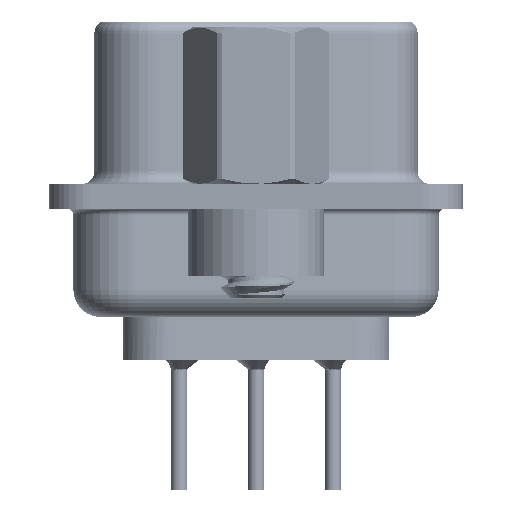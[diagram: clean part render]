
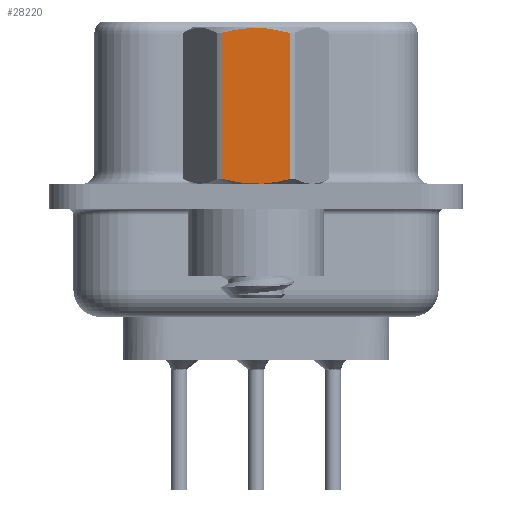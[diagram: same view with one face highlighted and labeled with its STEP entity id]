
A CAD part, left-side view. The second image highlights one B-rep face of the part: STEP entity #28220.
In plain terms, the highlighted planar face has unit normal (-1, 0, 0).
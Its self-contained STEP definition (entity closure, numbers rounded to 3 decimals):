
#46 = DIRECTION ( 'NONE',  ( 0., 0., -1. ) ) ;
#1586 = CARTESIAN_POINT ( 'NONE',  ( -2.381, 0.215, 6.232 ) ) ;
#3322 = VERTEX_POINT ( 'NONE', #21948 ) ;
#4261 = CARTESIAN_POINT ( 'NONE',  ( -2.381, 0.215, 0.468 ) ) ;
#6745 = CARTESIAN_POINT ( 'NONE',  ( -2.381, 1.273, 0.652 ) ) ;
#6927 = ORIENTED_EDGE ( 'NONE', *, *, #16355, .T. ) ;
#8190 = CARTESIAN_POINT ( 'NONE',  ( -2.381, 1.273, 6.048 ) ) ;
#8741 = LINE ( 'NONE', #14932, #22452 ) ;
#8798 = CARTESIAN_POINT ( 'NONE',  ( -2.381, 0.853, 6.151 ) ) ;
#10250 = CARTESIAN_POINT ( 'NONE',  ( -2.381, -1.273, 0.652 ) ) ;
#10459 = CARTESIAN_POINT ( 'NONE',  ( -2.381, -0.432, 0.485 ) ) ;
#10868 = CARTESIAN_POINT ( 'NONE',  ( -2.381, 1.065, 0.596 ) ) ;
#11129 = B_SPLINE_CURVE_WITH_KNOTS ( 'NONE', 3,
 ( #6745, #10868, #26337, #38489, #4261, #26128, #10459, #34998, #19337, #10250 ),
 .UNSPECIFIED., .F., .F.,
 ( 4, 2, 2, 2, 4 ),
 ( 0.003, 0.003, 0.004, 0.004, 0.005 ),
 .UNSPECIFIED. ) ;
#11699 = FACE_OUTER_BOUND ( 'NONE', #35062, .T. ) ;
#12107 = PLANE ( 'NONE',  #18965 ) ;
#13501 = CARTESIAN_POINT ( 'NONE',  ( -2.381, -1.273, 3.792 ) ) ;
#14485 = B_SPLINE_CURVE_WITH_KNOTS ( 'NONE', 3,
 ( #23662, #23869, #37036, #24078, #30651, #1586, #27147, #8798, #18285, #8190 ),
 .UNSPECIFIED., .F., .F.,
 ( 4, 2, 2, 2, 4 ),
 ( 0.001, 0.002, 0.002, 0.003, 0.004 ),
 .UNSPECIFIED. ) ;
#14932 = CARTESIAN_POINT ( 'NONE',  ( -2.381, 1.273, 3.792 ) ) ;
#15634 = EDGE_CURVE ( 'NONE', #16722, #33595, #11129, .T. ) ;
#16355 = EDGE_CURVE ( 'NONE', #35478, #16722, #8741, .T. ) ;
#16722 = VERTEX_POINT ( 'NONE', #19343 ) ;
#17099 = EDGE_CURVE ( 'NONE', #3322, #35478, #14485, .T. ) ;
#18285 = CARTESIAN_POINT ( 'NONE',  ( -2.381, 1.065, 6.104 ) ) ;
#18604 = VECTOR ( 'NONE', #35342, 1000. ) ;
#18965 = AXIS2_PLACEMENT_3D ( 'NONE', #21388, #24688, #33959 ) ;
#19337 = CARTESIAN_POINT ( 'NONE',  ( -2.381, -1.066, 0.596 ) ) ;
#19343 = CARTESIAN_POINT ( 'NONE',  ( -2.381, 1.273, 0.652 ) ) ;
#19867 = ORIENTED_EDGE ( 'NONE', *, *, #17099, .T. ) ;
#21388 = CARTESIAN_POINT ( 'NONE',  ( -2.381, 1.375, -3.75 ) ) ;
#21948 = CARTESIAN_POINT ( 'NONE',  ( -2.381, -1.273, 6.048 ) ) ;
#22452 = VECTOR ( 'NONE', #46, 1000. ) ;
#23662 = CARTESIAN_POINT ( 'NONE',  ( -2.381, -1.273, 6.048 ) ) ;
#23869 = CARTESIAN_POINT ( 'NONE',  ( -2.381, -1.066, 6.104 ) ) ;
#24012 = EDGE_CURVE ( 'NONE', #33595, #3322, #28966, .T. ) ;
#24078 = CARTESIAN_POINT ( 'NONE',  ( -2.381, -0.432, 6.215 ) ) ;
#24688 = DIRECTION ( 'NONE',  ( -1., 0., 0. ) ) ;
#26128 = CARTESIAN_POINT ( 'NONE',  ( -2.381, -0.215, 0.468 ) ) ;
#26337 = CARTESIAN_POINT ( 'NONE',  ( -2.381, 0.853, 0.549 ) ) ;
#27147 = CARTESIAN_POINT ( 'NONE',  ( -2.381, 0.428, 6.215 ) ) ;
#28220 = ADVANCED_FACE ( 'NONE', ( #11699 ), #12107, .T. ) ;
#28748 = CARTESIAN_POINT ( 'NONE',  ( -2.381, 1.273, 6.048 ) ) ;
#28966 = LINE ( 'NONE', #13501, #18604 ) ;
#30651 = CARTESIAN_POINT ( 'NONE',  ( -2.381, -0.215, 6.232 ) ) ;
#33421 = CARTESIAN_POINT ( 'NONE',  ( -2.381, -1.273, 0.652 ) ) ;
#33595 = VERTEX_POINT ( 'NONE', #33421 ) ;
#33959 = DIRECTION ( 'NONE',  ( 0., -1., 0. ) ) ;
#34998 = CARTESIAN_POINT ( 'NONE',  ( -2.381, -0.858, 0.55 ) ) ;
#35062 = EDGE_LOOP ( 'NONE', ( #39755, #38770, #19867, #6927 ) ) ;
#35342 = DIRECTION ( 'NONE',  ( 0., 0., 1. ) ) ;
#35478 = VERTEX_POINT ( 'NONE', #28748 ) ;
#37036 = CARTESIAN_POINT ( 'NONE',  ( -2.381, -0.858, 6.15 ) ) ;
#38489 = CARTESIAN_POINT ( 'NONE',  ( -2.381, 0.428, 0.485 ) ) ;
#38770 = ORIENTED_EDGE ( 'NONE', *, *, #24012, .T. ) ;
#39755 = ORIENTED_EDGE ( 'NONE', *, *, #15634, .T. ) ;
